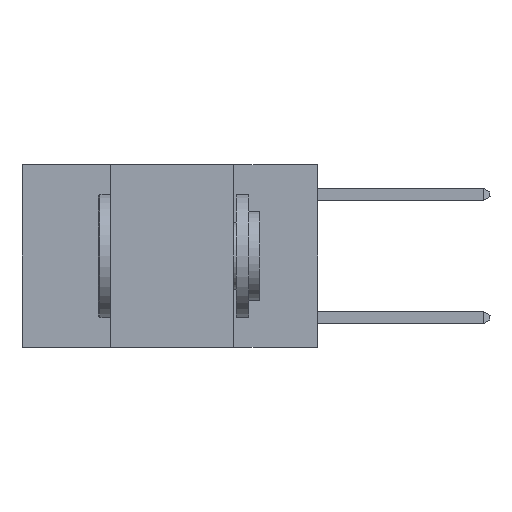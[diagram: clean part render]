
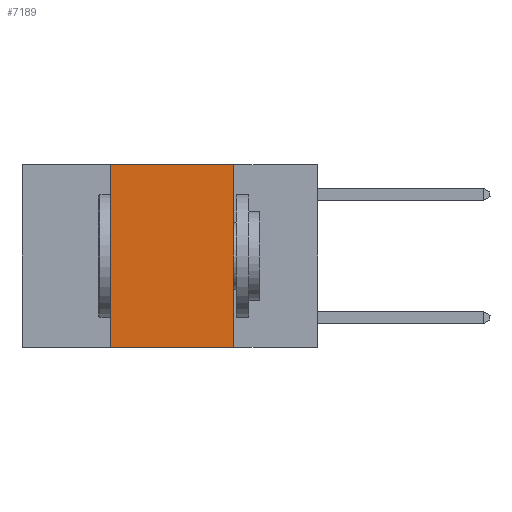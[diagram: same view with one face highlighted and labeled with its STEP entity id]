
A CAD part, left-side view. The second image highlights one B-rep face of the part: STEP entity #7189.
In plain terms, the highlighted planar face has unit normal (-1, 0, 0).
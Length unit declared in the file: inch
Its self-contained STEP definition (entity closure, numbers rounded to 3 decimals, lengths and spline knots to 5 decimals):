
#916 = DIRECTION ( 'NONE',  ( 0., -1., 0. ) ) ;
#1642 = LINE ( 'NONE', #6159, #8592 ) ;
#1883 = EDGE_CURVE ( 'NONE', #15653, #6585, #8356, .T. ) ;
#3161 = CARTESIAN_POINT ( 'NONE',  ( 0., 0.6, 0. ) ) ;
#3787 = ORIENTED_EDGE ( 'NONE', *, *, #1883, .F. ) ;
#4855 = CARTESIAN_POINT ( 'NONE',  ( 0., 0.17, 0. ) ) ;
#5627 = VECTOR ( 'NONE', #916, 39.37008 ) ;
#5710 = DIRECTION ( 'NONE',  ( 0., -1., 0. ) ) ;
#6159 = CARTESIAN_POINT ( 'NONE',  ( 0., 0.42, 0. ) ) ;
#6333 = VECTOR ( 'NONE', #5710, 39.37008 ) ;
#6462 = CARTESIAN_POINT ( 'NONE',  ( 0., 0.17, -0.37 ) ) ;
#6585 = VERTEX_POINT ( 'NONE', #4855 ) ;
#7189 = ADVANCED_FACE ( 'NONE', ( #13724 ), #7396, .F. ) ;
#7396 = PLANE ( 'NONE',  #8258 ) ;
#7480 = DIRECTION ( 'NONE',  ( 1., 0., 0. ) ) ;
#7784 = EDGE_CURVE ( 'NONE', #6585, #12917, #7958, .T. ) ;
#7958 = LINE ( 'NONE', #11265, #16485 ) ;
#8137 = ORIENTED_EDGE ( 'NONE', *, *, #19454, .F. ) ;
#8258 = AXIS2_PLACEMENT_3D ( 'NONE', #3161, #7480, #9286 ) ;
#8356 = LINE ( 'NONE', #17911, #5627 ) ;
#8521 = ORIENTED_EDGE ( 'NONE', *, *, #7784, .F. ) ;
#8592 = VECTOR ( 'NONE', #12301, 39.37008 ) ;
#9286 = DIRECTION ( 'NONE',  ( 0., 0., -1. ) ) ;
#10130 = LINE ( 'NONE', #13449, #6333 ) ;
#10729 = CARTESIAN_POINT ( 'NONE',  ( 0., 0.42, -0.37 ) ) ;
#11265 = CARTESIAN_POINT ( 'NONE',  ( 0., 0.17, 0. ) ) ;
#12301 = DIRECTION ( 'NONE',  ( 0., 0., 1. ) ) ;
#12917 = VERTEX_POINT ( 'NONE', #6462 ) ;
#13116 = EDGE_LOOP ( 'NONE', ( #8521, #3787, #8137, #19158 ) ) ;
#13449 = CARTESIAN_POINT ( 'NONE',  ( 0., 0.6, -0.37 ) ) ;
#13724 = FACE_OUTER_BOUND ( 'NONE', #13116, .T. ) ;
#15653 = VERTEX_POINT ( 'NONE', #16851 ) ;
#16485 = VECTOR ( 'NONE', #17401, 39.37008 ) ;
#16851 = CARTESIAN_POINT ( 'NONE',  ( 0., 0.42, 0. ) ) ;
#16983 = EDGE_CURVE ( 'NONE', #17156, #12917, #10130, .T. ) ;
#17156 = VERTEX_POINT ( 'NONE', #10729 ) ;
#17401 = DIRECTION ( 'NONE',  ( 0., 0., -1. ) ) ;
#17911 = CARTESIAN_POINT ( 'NONE',  ( 0., 0.6, 0. ) ) ;
#19158 = ORIENTED_EDGE ( 'NONE', *, *, #16983, .T. ) ;
#19454 = EDGE_CURVE ( 'NONE', #17156, #15653, #1642, .T. ) ;
